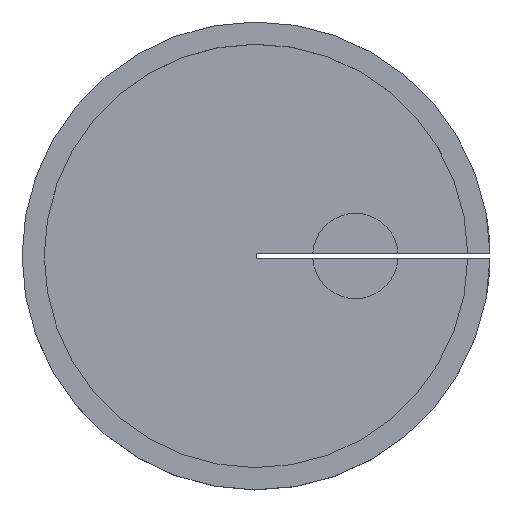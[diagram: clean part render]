
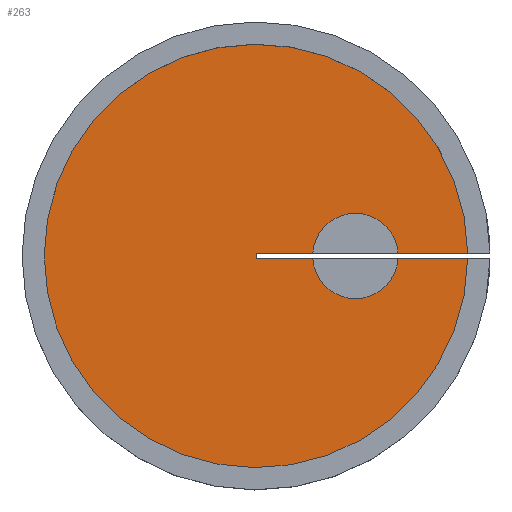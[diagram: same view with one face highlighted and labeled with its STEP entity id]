
A CAD part, top view. The second image highlights one B-rep face of the part: STEP entity #263.
In plain terms, the highlighted planar face has unit normal (0, 0, 1).
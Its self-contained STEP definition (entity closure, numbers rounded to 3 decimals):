
#26=CIRCLE('',#297,9.05);
#27=CIRCLE('',#299,1.825);
#28=CIRCLE('',#300,1.825);
#39=FACE_OUTER_BOUND('',#53,.T.);
#53=EDGE_LOOP('',(#221,#222,#223,#224,#225,#226,#227,#228));
#63=LINE('',#404,#89);
#67=LINE('',#412,#93);
#78=LINE('',#438,#104);
#82=LINE('',#446,#108);
#84=LINE('',#449,#110);
#89=VECTOR('',#323,10.);
#93=VECTOR('',#327,10.);
#104=VECTOR('',#348,10.);
#108=VECTOR('',#352,10.);
#110=VECTOR('',#356,10.);
#117=VERTEX_POINT('',#401);
#118=VERTEX_POINT('',#403);
#121=VERTEX_POINT('',#409);
#122=VERTEX_POINT('',#411);
#131=VERTEX_POINT('',#435);
#132=VERTEX_POINT('',#437);
#135=VERTEX_POINT('',#443);
#136=VERTEX_POINT('',#445);
#142=EDGE_CURVE('',#118,#117,#63,.F.);
#146=EDGE_CURVE('',#122,#121,#67,.F.);
#159=EDGE_CURVE('',#131,#132,#78,.T.);
#163=EDGE_CURVE('',#135,#136,#82,.T.);
#165=EDGE_CURVE('',#117,#136,#84,.T.);
#168=EDGE_CURVE('',#122,#131,#26,.F.);
#169=EDGE_CURVE('',#118,#121,#27,.T.);
#170=EDGE_CURVE('',#132,#135,#28,.T.);
#221=ORIENTED_EDGE('',*,*,#168,.F.);
#222=ORIENTED_EDGE('',*,*,#146,.T.);
#223=ORIENTED_EDGE('',*,*,#169,.F.);
#224=ORIENTED_EDGE('',*,*,#142,.T.);
#225=ORIENTED_EDGE('',*,*,#165,.T.);
#226=ORIENTED_EDGE('',*,*,#163,.F.);
#227=ORIENTED_EDGE('',*,*,#170,.F.);
#228=ORIENTED_EDGE('',*,*,#159,.F.);
#251=PLANE('',#298);
#263=ADVANCED_FACE('',(#39),#251,.F.);
#297=AXIS2_PLACEMENT_3D('',#454,#365,#366);
#298=AXIS2_PLACEMENT_3D('',#455,#367,#368);
#299=AXIS2_PLACEMENT_3D('',#456,#369,#370);
#300=AXIS2_PLACEMENT_3D('',#457,#371,#372);
#323=DIRECTION('',(1.,0.,0.));
#327=DIRECTION('',(1.,0.,0.));
#348=DIRECTION('',(-1.,0.,0.));
#352=DIRECTION('',(-1.,0.,0.));
#356=DIRECTION('',(0.,1.,0.));
#365=DIRECTION('center_axis',(0.,0.,
1.));
#366=DIRECTION('ref_axis',(-1.,0.,0.));
#367=DIRECTION('center_axis',(0.,0.,
-1.));
#368=DIRECTION('ref_axis',(-1.,0.,0.));
#369=DIRECTION('center_axis',(0.,0.,
1.));
#370=DIRECTION('ref_axis',(-1.,0.,0.));
#371=DIRECTION('center_axis',(0.,0.,
1.));
#372=DIRECTION('ref_axis',(-1.,0.,0.));
#401=CARTESIAN_POINT('',(-42.,-0.125,-12.));
#403=CARTESIAN_POINT('',(-39.571,-0.125,-12.));
#404=CARTESIAN_POINT('',(-42.,-0.125,-12.));
#409=CARTESIAN_POINT('',(-35.929,-0.125,-12.));
#411=CARTESIAN_POINT('',(-32.951,-0.125,-12.));
#412=CARTESIAN_POINT('',(-42.,-0.125,-12.));
#435=CARTESIAN_POINT('',(-32.951,0.125,-12.));
#437=CARTESIAN_POINT('',(-35.929,0.125,-12.));
#438=CARTESIAN_POINT('',(-37.002,0.125,-12.));
#443=CARTESIAN_POINT('',(-39.571,0.125,-12.));
#445=CARTESIAN_POINT('',(-42.,0.125,-12.));
#446=CARTESIAN_POINT('',(-37.002,0.125,-12.));
#449=CARTESIAN_POINT('',(-42.,0.125,-12.));
#454=CARTESIAN_POINT('Origin',(-42.,0.,-12.));
#455=CARTESIAN_POINT('Origin',(-42.,0.,-12.));
#456=CARTESIAN_POINT('Origin',(-37.75,0.,-12.));
#457=CARTESIAN_POINT('Origin',(-37.75,0.,-12.));
